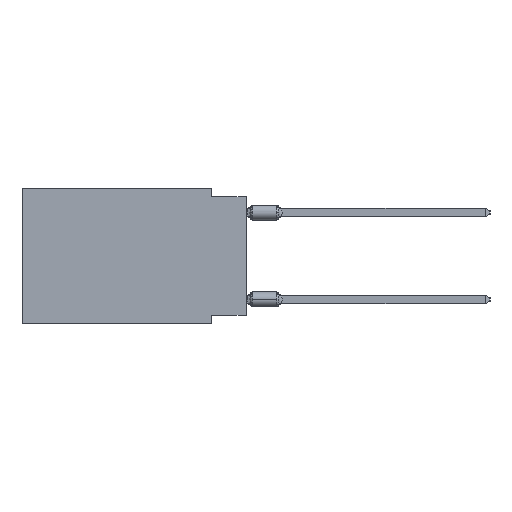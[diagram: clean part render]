
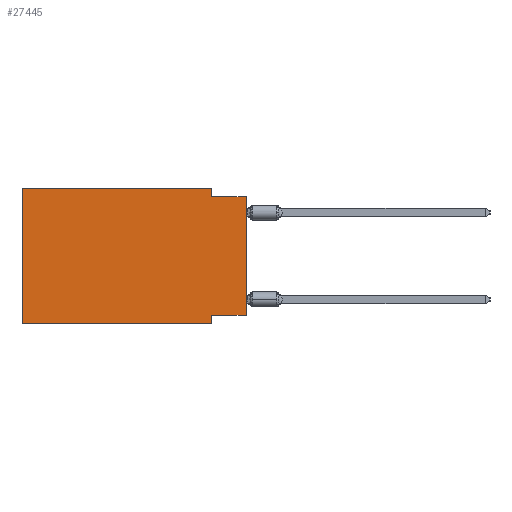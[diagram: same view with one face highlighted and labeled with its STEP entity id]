
A CAD part, left-side view. The second image highlights one B-rep face of the part: STEP entity #27445.
In plain terms, the highlighted planar face has unit normal (-1, 0, 0).
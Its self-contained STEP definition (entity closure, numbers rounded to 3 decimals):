
#260 = VERTEX_POINT ( 'NONE', #27440 ) ;
#5268 = VERTEX_POINT ( 'NONE', #57082 ) ;
#6874 = VECTOR ( 'NONE', #11313, 1000. ) ;
#8262 = CARTESIAN_POINT ( 'NONE',  ( 0., 0., -0.635 ) ) ;
#8961 = VECTOR ( 'NONE', #59816, 1000. ) ;
#11313 = DIRECTION ( 'NONE',  ( 0., -1., 0. ) ) ;
#11946 = VERTEX_POINT ( 'NONE', #53164 ) ;
#14043 = CARTESIAN_POINT ( 'NONE',  ( 0., 0., -9.271 ) ) ;
#14589 = ORIENTED_EDGE ( 'NONE', *, *, #23085, .F. ) ;
#15246 = VERTEX_POINT ( 'NONE', #28174 ) ;
#15377 = CARTESIAN_POINT ( 'NONE',  ( 0., 2.54, -9.271 ) ) ;
#15770 = ORIENTED_EDGE ( 'NONE', *, *, #21618, .T. ) ;
#17423 = AXIS2_PLACEMENT_3D ( 'NONE', #66103, #29844, #19255 ) ;
#17760 = DIRECTION ( 'NONE',  ( 0., 0., -1. ) ) ;
#18242 = PLANE ( 'NONE',  #17423 ) ;
#18436 = CARTESIAN_POINT ( 'NONE',  ( 0., 16.383, 0. ) ) ;
#19192 = LINE ( 'NONE', #14043, #20350 ) ;
#19255 = DIRECTION ( 'NONE',  ( 0., 0., -1. ) ) ;
#19645 = VECTOR ( 'NONE', #29450, 1000. ) ;
#20350 = VECTOR ( 'NONE', #55759, 1000. ) ;
#20662 = EDGE_CURVE ( 'NONE', #11946, #42891, #38345, .T. ) ;
#20824 = LINE ( 'NONE', #25271, #54172 ) ;
#21618 = EDGE_CURVE ( 'NONE', #260, #42891, #44814, .T. ) ;
#23085 = EDGE_CURVE ( 'NONE', #44083, #15246, #31522, .T. ) ;
#23230 = EDGE_CURVE ( 'NONE', #31583, #60001, #34153, .T. ) ;
#24485 = ORIENTED_EDGE ( 'NONE', *, *, #23230, .F. ) ;
#25271 = CARTESIAN_POINT ( 'NONE',  ( 0., 2.54, 0. ) ) ;
#27035 = LINE ( 'NONE', #63292, #6874 ) ;
#27440 = CARTESIAN_POINT ( 'NONE',  ( 0., 0., -9.271 ) ) ;
#27445 = ADVANCED_FACE ( 'NONE', ( #66432 ), #18242, .F. ) ;
#28174 = CARTESIAN_POINT ( 'NONE',  ( 0., 2.54, -9.906 ) ) ;
#29450 = DIRECTION ( 'NONE',  ( 0., -1., 0. ) ) ;
#29844 = DIRECTION ( 'NONE',  ( 1., 0., 0. ) ) ;
#30791 = ORIENTED_EDGE ( 'NONE', *, *, #31107, .F. ) ;
#31107 = EDGE_CURVE ( 'NONE', #5268, #11946, #20824, .T. ) ;
#31522 = LINE ( 'NONE', #43391, #59174 ) ;
#31583 = VERTEX_POINT ( 'NONE', #51526 ) ;
#34153 = LINE ( 'NONE', #18436, #8961 ) ;
#35941 = LINE ( 'NONE', #67087, #53807 ) ;
#36072 = VECTOR ( 'NONE', #50628, 1000. ) ;
#36610 = DIRECTION ( 'NONE',  ( 0., -1., 0. ) ) ;
#37471 = EDGE_LOOP ( 'NONE', ( #15770, #60487, #30791, #56613, #24485, #51063, #14589, #52798 ) ) ;
#38345 = LINE ( 'NONE', #8262, #19645 ) ;
#39693 = CARTESIAN_POINT ( 'NONE',  ( 0., 0., 0. ) ) ;
#40667 = DIRECTION ( 'NONE',  ( 0., 0., -1. ) ) ;
#42891 = VERTEX_POINT ( 'NONE', #47060 ) ;
#43391 = CARTESIAN_POINT ( 'NONE',  ( 0., 2.54, -9.906 ) ) ;
#44083 = VERTEX_POINT ( 'NONE', #15377 ) ;
#44814 = LINE ( 'NONE', #39693, #36072 ) ;
#45517 = EDGE_CURVE ( 'NONE', #260, #44083, #19192, .T. ) ;
#47060 = CARTESIAN_POINT ( 'NONE',  ( 0., 0., -0.635 ) ) ;
#50628 = DIRECTION ( 'NONE',  ( 0., 0., 1. ) ) ;
#50734 = CARTESIAN_POINT ( 'NONE',  ( 0., 16.383, 0. ) ) ;
#51063 = ORIENTED_EDGE ( 'NONE', *, *, #51192, .T. ) ;
#51192 = EDGE_CURVE ( 'NONE', #31583, #15246, #35941, .T. ) ;
#51526 = CARTESIAN_POINT ( 'NONE',  ( 0., 16.383, -9.906 ) ) ;
#52798 = ORIENTED_EDGE ( 'NONE', *, *, #45517, .F. ) ;
#53164 = CARTESIAN_POINT ( 'NONE',  ( 0., 2.54, -0.635 ) ) ;
#53807 = VECTOR ( 'NONE', #36610, 1000. ) ;
#54172 = VECTOR ( 'NONE', #40667, 1000. ) ;
#55759 = DIRECTION ( 'NONE',  ( 0., 1., 0. ) ) ;
#56613 = ORIENTED_EDGE ( 'NONE', *, *, #61150, .F. ) ;
#57082 = CARTESIAN_POINT ( 'NONE',  ( 0., 2.54, 0. ) ) ;
#59174 = VECTOR ( 'NONE', #17760, 1000. ) ;
#59816 = DIRECTION ( 'NONE',  ( 0., 0., 1. ) ) ;
#60001 = VERTEX_POINT ( 'NONE', #50734 ) ;
#60487 = ORIENTED_EDGE ( 'NONE', *, *, #20662, .F. ) ;
#61150 = EDGE_CURVE ( 'NONE', #60001, #5268, #27035, .T. ) ;
#63292 = CARTESIAN_POINT ( 'NONE',  ( 0., 16.383, 0. ) ) ;
#66103 = CARTESIAN_POINT ( 'NONE',  ( 0., 16.383, 0. ) ) ;
#66432 = FACE_OUTER_BOUND ( 'NONE', #37471, .T. ) ;
#67087 = CARTESIAN_POINT ( 'NONE',  ( 0., 16.383, -9.906 ) ) ;
